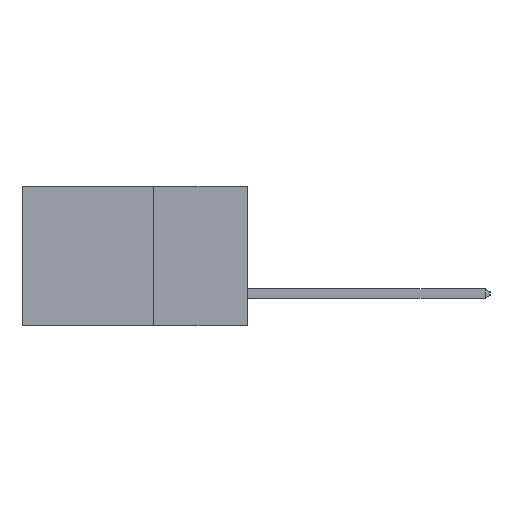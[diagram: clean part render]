
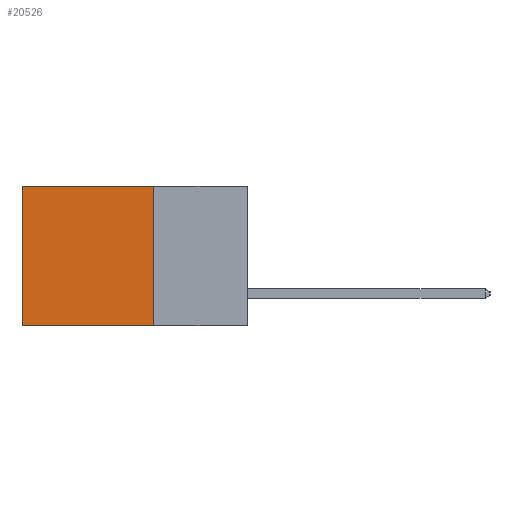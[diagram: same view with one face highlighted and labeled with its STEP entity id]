
A CAD part, left-side view. The second image highlights one B-rep face of the part: STEP entity #20526.
In plain terms, the highlighted planar face has unit normal (-1, 0, 0).
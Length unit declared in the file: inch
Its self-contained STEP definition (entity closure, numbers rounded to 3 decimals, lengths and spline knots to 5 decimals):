
#223 = DIRECTION ( 'NONE',  ( 0., 0., -1. ) ) ;
#1636 = CARTESIAN_POINT ( 'NONE',  ( 0.298, 0.25, 0. ) ) ;
#4196 = DIRECTION ( 'NONE',  ( 0., 0., -1. ) ) ;
#5042 = VERTEX_POINT ( 'NONE', #17176 ) ;
#5975 = DIRECTION ( 'NONE',  ( 0., 0., -1. ) ) ;
#7577 = VECTOR ( 'NONE', #30570, 39.37008 ) ;
#8060 = CARTESIAN_POINT ( 'NONE',  ( 0.298, 0.6, -0.37 ) ) ;
#8329 = CARTESIAN_POINT ( 'NONE',  ( 0.298, 0.25, -0.37 ) ) ;
#10229 = VERTEX_POINT ( 'NONE', #8060 ) ;
#10386 = CARTESIAN_POINT ( 'NONE',  ( 0.298, 0.25, -0.37 ) ) ;
#10824 = VERTEX_POINT ( 'NONE', #17874 ) ;
#12703 = PLANE ( 'NONE',  #23202 ) ;
#12804 = LINE ( 'NONE', #1636, #17851 ) ;
#15137 = CARTESIAN_POINT ( 'NONE',  ( 0.298, 0.25, 0. ) ) ;
#15252 = DIRECTION ( 'NONE',  ( 1., 0., 0. ) ) ;
#17176 = CARTESIAN_POINT ( 'NONE',  ( 0.298, 0.6, 0. ) ) ;
#17621 = VECTOR ( 'NONE', #18283, 39.37008 ) ;
#17851 = VECTOR ( 'NONE', #4196, 39.37008 ) ;
#17874 = CARTESIAN_POINT ( 'NONE',  ( 0.298, 0.25, 0. ) ) ;
#18283 = DIRECTION ( 'NONE',  ( 0., 1., 0. ) ) ;
#18344 = CARTESIAN_POINT ( 'NONE',  ( 0.298, 0.6, 0. ) ) ;
#20033 = EDGE_CURVE ( 'NONE', #29745, #10229, #24892, .T. ) ;
#20526 = ADVANCED_FACE ( 'NONE', ( #28196 ), #12703, .F. ) ;
#22659 = EDGE_LOOP ( 'NONE', ( #22806, #24385, #27732, #27295 ) ) ;
#22806 = ORIENTED_EDGE ( 'NONE', *, *, #31121, .T. ) ;
#23202 = AXIS2_PLACEMENT_3D ( 'NONE', #15137, #15252, #223 ) ;
#24385 = ORIENTED_EDGE ( 'NONE', *, *, #20033, .F. ) ;
#24892 = LINE ( 'NONE', #8329, #17621 ) ;
#25494 = LINE ( 'NONE', #18344, #30343 ) ;
#25872 = CARTESIAN_POINT ( 'NONE',  ( 0.298, 0.25, 0. ) ) ;
#27160 = LINE ( 'NONE', #25872, #7577 ) ;
#27295 = ORIENTED_EDGE ( 'NONE', *, *, #28625, .T. ) ;
#27732 = ORIENTED_EDGE ( 'NONE', *, *, #31303, .F. ) ;
#28196 = FACE_OUTER_BOUND ( 'NONE', #22659, .T. ) ;
#28625 = EDGE_CURVE ( 'NONE', #10824, #5042, #27160, .T. ) ;
#29745 = VERTEX_POINT ( 'NONE', #10386 ) ;
#30343 = VECTOR ( 'NONE', #5975, 39.37008 ) ;
#30570 = DIRECTION ( 'NONE',  ( 0., 1., 0. ) ) ;
#31121 = EDGE_CURVE ( 'NONE', #5042, #10229, #25494, .T. ) ;
#31303 = EDGE_CURVE ( 'NONE', #10824, #29745, #12804, .T. ) ;
